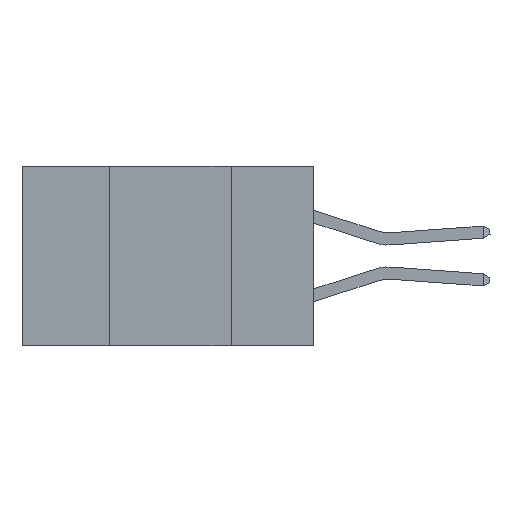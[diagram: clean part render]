
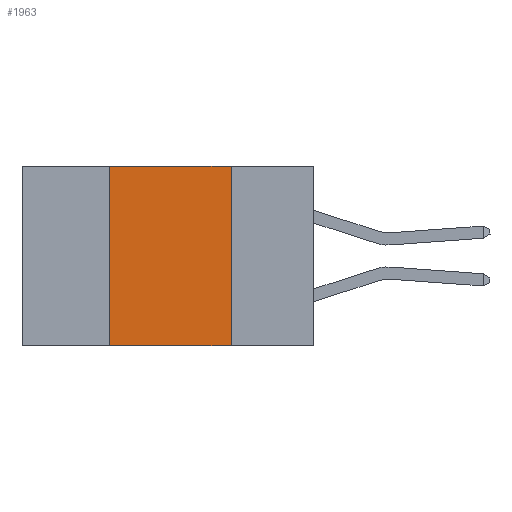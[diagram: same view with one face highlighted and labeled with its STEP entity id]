
A CAD part, left-side view. The second image highlights one B-rep face of the part: STEP entity #1963.
In plain terms, the highlighted planar face has unit normal (-1, 0, 0).
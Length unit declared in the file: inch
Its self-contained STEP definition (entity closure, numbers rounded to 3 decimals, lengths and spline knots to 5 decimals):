
#246 = FACE_OUTER_BOUND ( 'NONE', #5364, .T. ) ;
#821 = VERTEX_POINT ( 'NONE', #1581 ) ;
#1055 = DIRECTION ( 'NONE',  ( 0., -1., 0. ) ) ;
#1581 = CARTESIAN_POINT ( 'NONE',  ( 0., 0.42, -0.37 ) ) ;
#1791 = DIRECTION ( 'NONE',  ( 1., 0., 0. ) ) ;
#1941 = LINE ( 'NONE', #4151, #13817 ) ;
#1963 = ADVANCED_FACE ( 'NONE', ( #246 ), #14062, .F. ) ;
#2244 = VECTOR ( 'NONE', #5771, 39.37008 ) ;
#2509 = CARTESIAN_POINT ( 'NONE',  ( 0., 0.6, -0.37 ) ) ;
#2582 = ORIENTED_EDGE ( 'NONE', *, *, #4414, .F. ) ;
#2763 = DIRECTION ( 'NONE',  ( 0., -1., 0. ) ) ;
#3020 = CARTESIAN_POINT ( 'NONE',  ( 0., 0.6, 0. ) ) ;
#4151 = CARTESIAN_POINT ( 'NONE',  ( 0., 0.17, 0. ) ) ;
#4332 = VECTOR ( 'NONE', #2763, 39.37008 ) ;
#4414 = EDGE_CURVE ( 'NONE', #15875, #5408, #13424, .T. ) ;
#4550 = CARTESIAN_POINT ( 'NONE',  ( 0., 0.42, 0. ) ) ;
#4587 = ORIENTED_EDGE ( 'NONE', *, *, #11104, .F. ) ;
#4719 = EDGE_CURVE ( 'NONE', #821, #15875, #14478, .T. ) ;
#4844 = ORIENTED_EDGE ( 'NONE', *, *, #4917, .T. ) ;
#4917 = EDGE_CURVE ( 'NONE', #821, #7466, #8865, .T. ) ;
#5364 = EDGE_LOOP ( 'NONE', ( #4587, #2582, #15211, #4844 ) ) ;
#5408 = VERTEX_POINT ( 'NONE', #11113 ) ;
#5771 = DIRECTION ( 'NONE',  ( 0., 0., 1. ) ) ;
#6586 = DIRECTION ( 'NONE',  ( 0., 0., -1. ) ) ;
#7466 = VERTEX_POINT ( 'NONE', #14568 ) ;
#8865 = LINE ( 'NONE', #2509, #4332 ) ;
#10264 = CARTESIAN_POINT ( 'NONE',  ( 0., 0.42, 0. ) ) ;
#11104 = EDGE_CURVE ( 'NONE', #5408, #7466, #1941, .T. ) ;
#11113 = CARTESIAN_POINT ( 'NONE',  ( 0., 0.17, 0. ) ) ;
#11724 = DIRECTION ( 'NONE',  ( 0., 0., -1. ) ) ;
#12211 = CARTESIAN_POINT ( 'NONE',  ( 0., 0.6, 0. ) ) ;
#12355 = VECTOR ( 'NONE', #1055, 39.37008 ) ;
#12592 = AXIS2_PLACEMENT_3D ( 'NONE', #3020, #1791, #11724 ) ;
#13424 = LINE ( 'NONE', #12211, #12355 ) ;
#13817 = VECTOR ( 'NONE', #6586, 39.37008 ) ;
#14062 = PLANE ( 'NONE',  #12592 ) ;
#14478 = LINE ( 'NONE', #4550, #2244 ) ;
#14568 = CARTESIAN_POINT ( 'NONE',  ( 0., 0.17, -0.37 ) ) ;
#15211 = ORIENTED_EDGE ( 'NONE', *, *, #4719, .F. ) ;
#15875 = VERTEX_POINT ( 'NONE', #10264 ) ;
